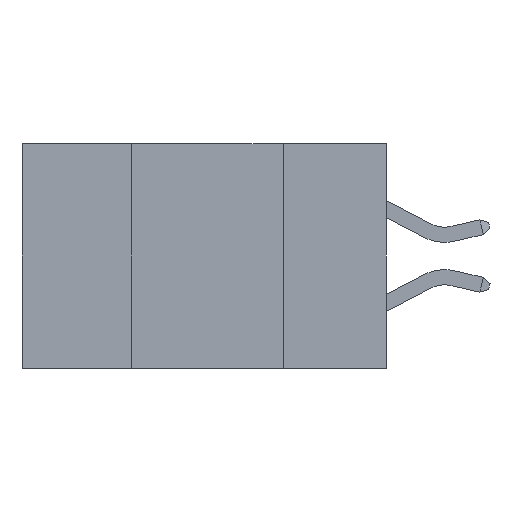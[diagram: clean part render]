
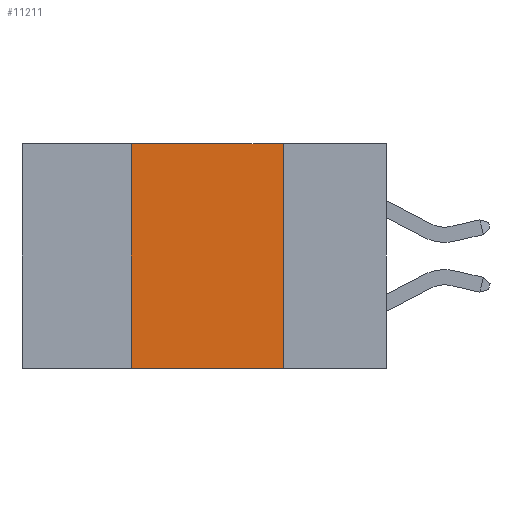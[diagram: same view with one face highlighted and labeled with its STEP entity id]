
A CAD part, left-side view. The second image highlights one B-rep face of the part: STEP entity #11211.
In plain terms, the highlighted planar face has unit normal (-1, 0, 0).
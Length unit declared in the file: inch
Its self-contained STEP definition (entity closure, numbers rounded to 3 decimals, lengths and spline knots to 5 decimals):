
#38 = CARTESIAN_POINT ( 'NONE',  ( 0., 0.42, 0. ) ) ;
#503 = EDGE_CURVE ( 'NONE', #11398, #2798, #12017, .T. ) ;
#532 = VECTOR ( 'NONE', #7814, 39.37008 ) ;
#1157 = VERTEX_POINT ( 'NONE', #6401 ) ;
#2728 = CARTESIAN_POINT ( 'NONE',  ( 0., 0.42, -0.37 ) ) ;
#2798 = VERTEX_POINT ( 'NONE', #13005 ) ;
#3028 = FACE_OUTER_BOUND ( 'NONE', #6393, .T. ) ;
#3692 = DIRECTION ( 'NONE',  ( 0., -1., 0. ) ) ;
#3731 = VECTOR ( 'NONE', #3692, 39.37008 ) ;
#3914 = VERTEX_POINT ( 'NONE', #38 ) ;
#4131 = DIRECTION ( 'NONE',  ( 0., -1., 0. ) ) ;
#4145 = DIRECTION ( 'NONE',  ( 0., 0., -1. ) ) ;
#4407 = ORIENTED_EDGE ( 'NONE', *, *, #8556, .F. ) ;
#5583 = DIRECTION ( 'NONE',  ( 1., 0., 0. ) ) ;
#6393 = EDGE_LOOP ( 'NONE', ( #4407, #8063, #8184, #7850 ) ) ;
#6401 = CARTESIAN_POINT ( 'NONE',  ( 0., 0.17, 0. ) ) ;
#6749 = CARTESIAN_POINT ( 'NONE',  ( 0., 0.42, -0.37 ) ) ;
#6777 = LINE ( 'NONE', #9372, #12612 ) ;
#7118 = LINE ( 'NONE', #12462, #7452 ) ;
#7452 = VECTOR ( 'NONE', #4145, 39.37008 ) ;
#7684 = PLANE ( 'NONE',  #12814 ) ;
#7814 = DIRECTION ( 'NONE',  ( 0., 0., 1. ) ) ;
#7850 = ORIENTED_EDGE ( 'NONE', *, *, #503, .T. ) ;
#7966 = LINE ( 'NONE', #6749, #532 ) ;
#8063 = ORIENTED_EDGE ( 'NONE', *, *, #9242, .F. ) ;
#8184 = ORIENTED_EDGE ( 'NONE', *, *, #11288, .F. ) ;
#8556 = EDGE_CURVE ( 'NONE', #1157, #2798, #7118, .T. ) ;
#9242 = EDGE_CURVE ( 'NONE', #3914, #1157, #6777, .T. ) ;
#9372 = CARTESIAN_POINT ( 'NONE',  ( 0., 0.6, 0. ) ) ;
#11211 = ADVANCED_FACE ( 'NONE', ( #3028 ), #7684, .F. ) ;
#11288 = EDGE_CURVE ( 'NONE', #11398, #3914, #7966, .T. ) ;
#11398 = VERTEX_POINT ( 'NONE', #2728 ) ;
#11818 = CARTESIAN_POINT ( 'NONE',  ( 0., 0.6, 0. ) ) ;
#12017 = LINE ( 'NONE', #13030, #3731 ) ;
#12462 = CARTESIAN_POINT ( 'NONE',  ( 0., 0.17, -0.37 ) ) ;
#12612 = VECTOR ( 'NONE', #4131, 39.37008 ) ;
#12814 = AXIS2_PLACEMENT_3D ( 'NONE', #11818, #5583, #12853 ) ;
#12853 = DIRECTION ( 'NONE',  ( 0., 0., -1. ) ) ;
#13005 = CARTESIAN_POINT ( 'NONE',  ( 0., 0.17, -0.37 ) ) ;
#13030 = CARTESIAN_POINT ( 'NONE',  ( 0., 0.6, -0.37 ) ) ;
